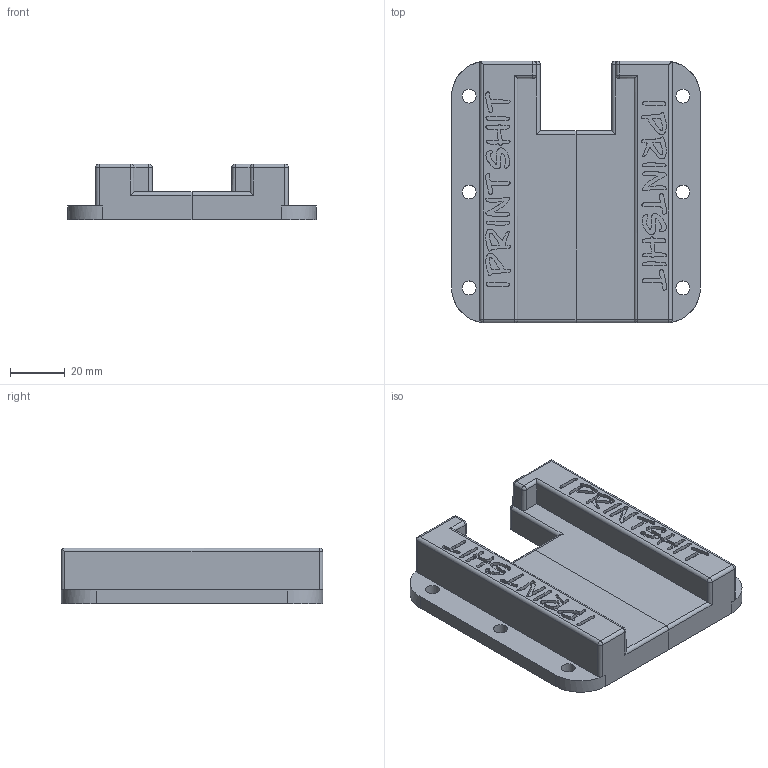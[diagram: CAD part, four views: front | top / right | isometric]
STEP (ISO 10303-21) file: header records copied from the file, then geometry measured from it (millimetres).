
FILE_DESCRIPTION(/* description */ (''),/* implementation_level */ '2;1');
FILE_NAME(/* name */ 'Grip n Rip Glockofsky.step',/* time_stamp */ '2022-04-04T10:13:42-07:00',/* author */ (''),/* organization */ (''),/* preprocessor_version */ 'ST-DEVELOPER v18.1',/* originating_system */ 'Autodesk Translation Framework v10.14.0.1471',/* authorisation */ '');
FILE_SCHEMA (('AUTOMOTIVE_DESIGN { 1 0 10303 214 3 1 1 }'));
Length unit declared in the file: inch
Products named in the file (1): Quickdraw V3
Bounding box: 90.54 x 95.25 x 20.32 mm (x, y, z)
Volume: 66349.1 mm3; surface area: 30152.9 mm2
Topology: 2 solids, 2 shells, 522 faces, 1434 edges, 940 vertices
Faces by surface type: bspline 354, plane 112, cylinder 46, sphere 10
Full cylindrical faces by diameter (mm): 5.08 x6, 33.02 x4
Entity records: 17344 total; most frequent: CARTESIAN_POINT 7501, ORIENTED_EDGE 2860, EDGE_CURVE 1430, DIRECTION 1146, VERTEX_POINT 940, LINE 632, VECTOR 632, EDGE_LOOP 562
